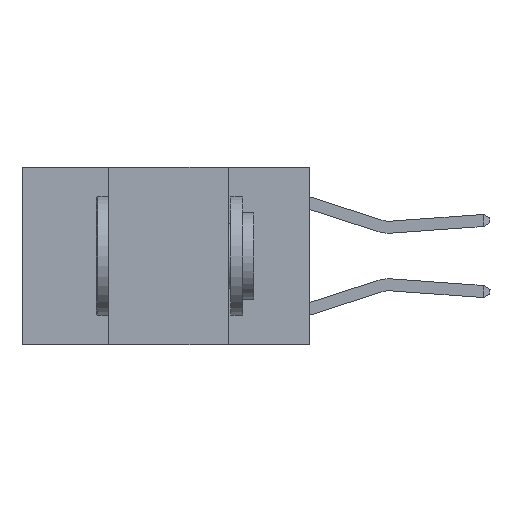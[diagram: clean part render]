
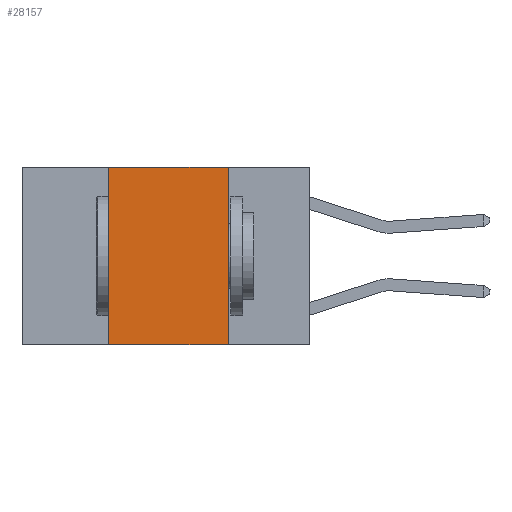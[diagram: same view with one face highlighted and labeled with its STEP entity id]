
A CAD part, left-side view. The second image highlights one B-rep face of the part: STEP entity #28157.
In plain terms, the highlighted planar face has unit normal (-1, 0, 0).
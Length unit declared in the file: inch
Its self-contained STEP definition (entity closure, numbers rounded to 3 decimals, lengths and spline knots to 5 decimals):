
#663 = LINE ( 'NONE', #3275, #6595 ) ;
#2665 = VECTOR ( 'NONE', #23156, 39.37008 ) ;
#3275 = CARTESIAN_POINT ( 'NONE',  ( 0., 0.6, 0. ) ) ;
#4325 = EDGE_CURVE ( 'NONE', #7430, #22271, #663, .T. ) ;
#4681 = DIRECTION ( 'NONE',  ( 1., 0., 0. ) ) ;
#4730 = CARTESIAN_POINT ( 'NONE',  ( 0., 0.17, 0. ) ) ;
#6595 = VECTOR ( 'NONE', #18513, 39.37008 ) ;
#7430 = VERTEX_POINT ( 'NONE', #11849 ) ;
#8983 = VECTOR ( 'NONE', #11555, 39.37008 ) ;
#10567 = CARTESIAN_POINT ( 'NONE',  ( 0., 0.6, -0.37 ) ) ;
#11555 = DIRECTION ( 'NONE',  ( 0., 0., 1. ) ) ;
#11849 = CARTESIAN_POINT ( 'NONE',  ( 0., 0.42, 0. ) ) ;
#13161 = VERTEX_POINT ( 'NONE', #30165 ) ;
#13904 = EDGE_CURVE ( 'NONE', #22271, #16417, #26592, .T. ) ;
#16417 = VERTEX_POINT ( 'NONE', #21892 ) ;
#16515 = ORIENTED_EDGE ( 'NONE', *, *, #13904, .F. ) ;
#16639 = CARTESIAN_POINT ( 'NONE',  ( 0., 0.42, 0. ) ) ;
#16807 = VECTOR ( 'NONE', #29560, 39.37008 ) ;
#18513 = DIRECTION ( 'NONE',  ( 0., -1., 0. ) ) ;
#19544 = AXIS2_PLACEMENT_3D ( 'NONE', #27124, #4681, #30253 ) ;
#20212 = LINE ( 'NONE', #10567, #2665 ) ;
#21892 = CARTESIAN_POINT ( 'NONE',  ( 0., 0.17, -0.37 ) ) ;
#22271 = VERTEX_POINT ( 'NONE', #4730 ) ;
#22700 = FACE_OUTER_BOUND ( 'NONE', #27317, .T. ) ;
#22795 = ORIENTED_EDGE ( 'NONE', *, *, #4325, .F. ) ;
#23156 = DIRECTION ( 'NONE',  ( 0., -1., 0. ) ) ;
#24377 = EDGE_CURVE ( 'NONE', #13161, #7430, #31070, .T. ) ;
#24648 = EDGE_CURVE ( 'NONE', #13161, #16417, #20212, .T. ) ;
#24668 = PLANE ( 'NONE',  #19544 ) ;
#26592 = LINE ( 'NONE', #27082, #16807 ) ;
#27082 = CARTESIAN_POINT ( 'NONE',  ( 0., 0.17, 0. ) ) ;
#27124 = CARTESIAN_POINT ( 'NONE',  ( 0., 0.6, 0. ) ) ;
#27317 = EDGE_LOOP ( 'NONE', ( #16515, #22795, #27727, #27876 ) ) ;
#27727 = ORIENTED_EDGE ( 'NONE', *, *, #24377, .F. ) ;
#27876 = ORIENTED_EDGE ( 'NONE', *, *, #24648, .T. ) ;
#28157 = ADVANCED_FACE ( 'NONE', ( #22700 ), #24668, .F. ) ;
#29560 = DIRECTION ( 'NONE',  ( 0., 0., -1. ) ) ;
#30165 = CARTESIAN_POINT ( 'NONE',  ( 0., 0.42, -0.37 ) ) ;
#30253 = DIRECTION ( 'NONE',  ( 0., 0., -1. ) ) ;
#31070 = LINE ( 'NONE', #16639, #8983 ) ;
